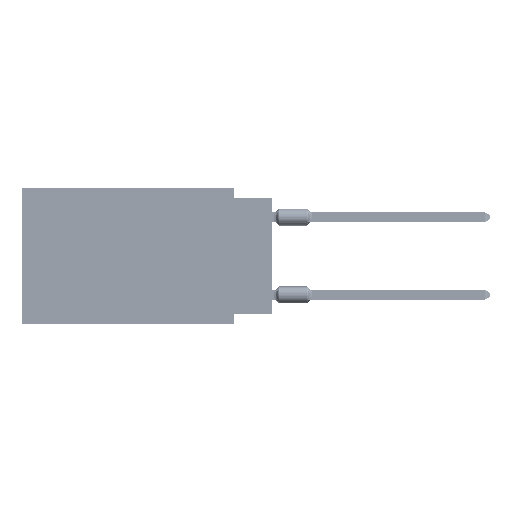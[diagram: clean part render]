
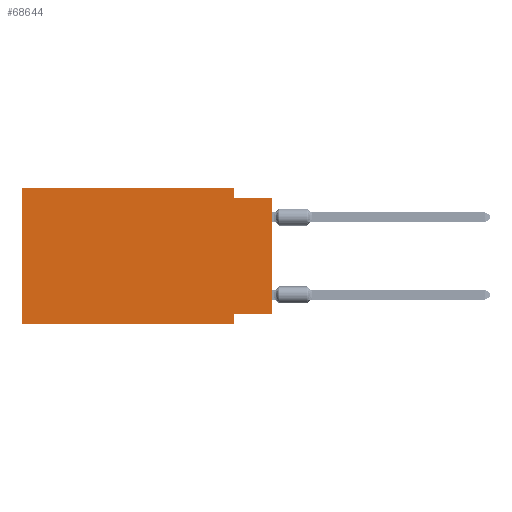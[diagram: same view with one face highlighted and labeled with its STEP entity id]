
A CAD part, left-side view. The second image highlights one B-rep face of the part: STEP entity #68644.
In plain terms, the highlighted planar face has unit normal (-1, 0, 0).
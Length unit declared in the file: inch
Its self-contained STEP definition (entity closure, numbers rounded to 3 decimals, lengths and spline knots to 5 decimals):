
#1004 = DIRECTION ( 'NONE',  ( 0., 0., 1. ) ) ;
#1669 = VECTOR ( 'NONE', #36369, 39.37008 ) ;
#2218 = EDGE_CURVE ( 'NONE', #15262, #39468, #37346, .T. ) ;
#2413 = VECTOR ( 'NONE', #67750, 39.37008 ) ;
#2530 = LINE ( 'NONE', #11505, #83795 ) ;
#3636 = VECTOR ( 'NONE', #24250, 39.37008 ) ;
#4646 = VECTOR ( 'NONE', #72819, 39.37008 ) ;
#4656 = VERTEX_POINT ( 'NONE', #49987 ) ;
#7722 = CARTESIAN_POINT ( 'NONE',  ( 0., 0., -0.025 ) ) ;
#11505 = CARTESIAN_POINT ( 'NONE',  ( 0., 0.1, 0. ) ) ;
#15262 = VERTEX_POINT ( 'NONE', #28294 ) ;
#16620 = EDGE_CURVE ( 'NONE', #43277, #98050, #51358, .T. ) ;
#16876 = VERTEX_POINT ( 'NONE', #75508 ) ;
#17993 = CARTESIAN_POINT ( 'NONE',  ( 0., 0.645, 0. ) ) ;
#18963 = ORIENTED_EDGE ( 'NONE', *, *, #16620, .T. ) ;
#24250 = DIRECTION ( 'NONE',  ( 0., -1., 0. ) ) ;
#24276 = EDGE_LOOP ( 'NONE', ( #88267, #56653, #89453, #75175, #71357, #18963, #28171, #68368 ) ) ;
#27931 = LINE ( 'NONE', #80795, #4646 ) ;
#28171 = ORIENTED_EDGE ( 'NONE', *, *, #62878, .F. ) ;
#28294 = CARTESIAN_POINT ( 'NONE',  ( 0., 0.645, 0. ) ) ;
#29452 = CARTESIAN_POINT ( 'NONE',  ( 0., 0.1, -0.325 ) ) ;
#32954 = DIRECTION ( 'NONE',  ( 0., 0., -1. ) ) ;
#32984 = DIRECTION ( 'NONE',  ( 0., 0., -1. ) ) ;
#34914 = VERTEX_POINT ( 'NONE', #29452 ) ;
#34964 = CARTESIAN_POINT ( 'NONE',  ( 0., 0.1, 0. ) ) ;
#36369 = DIRECTION ( 'NONE',  ( 0., 1., 0. ) ) ;
#37346 = LINE ( 'NONE', #92174, #2413 ) ;
#38599 = EDGE_CURVE ( 'NONE', #16876, #40599, #75107, .T. ) ;
#39468 = VERTEX_POINT ( 'NONE', #34964 ) ;
#40599 = VERTEX_POINT ( 'NONE', #7722 ) ;
#43277 = VERTEX_POINT ( 'NONE', #55944 ) ;
#43360 = CARTESIAN_POINT ( 'NONE',  ( 0., 0., -0.325 ) ) ;
#44192 = CARTESIAN_POINT ( 'NONE',  ( 0., 0., -0.025 ) ) ;
#49382 = PLANE ( 'NONE',  #57606 ) ;
#49987 = CARTESIAN_POINT ( 'NONE',  ( 0., 0., -0.325 ) ) ;
#50325 = LINE ( 'NONE', #43360, #1669 ) ;
#51358 = LINE ( 'NONE', #67307, #3636 ) ;
#52248 = VECTOR ( 'NONE', #97023, 39.37008 ) ;
#53102 = DIRECTION ( 'NONE',  ( 0., 0., -1. ) ) ;
#53448 = EDGE_CURVE ( 'NONE', #39468, #16876, #2530, .T. ) ;
#55433 = VECTOR ( 'NONE', #53102, 39.37008 ) ;
#55944 = CARTESIAN_POINT ( 'NONE',  ( 0., 0.645, -0.35 ) ) ;
#56653 = ORIENTED_EDGE ( 'NONE', *, *, #38599, .F. ) ;
#57606 = AXIS2_PLACEMENT_3D ( 'NONE', #17993, #86795, #32954 ) ;
#62878 = EDGE_CURVE ( 'NONE', #34914, #98050, #77878, .T. ) ;
#64839 = FACE_OUTER_BOUND ( 'NONE', #24276, .T. ) ;
#65180 = CARTESIAN_POINT ( 'NONE',  ( 0., 0.1, -0.35 ) ) ;
#67307 = CARTESIAN_POINT ( 'NONE',  ( 0., 0.645, -0.35 ) ) ;
#67750 = DIRECTION ( 'NONE',  ( 0., -1., 0. ) ) ;
#68368 = ORIENTED_EDGE ( 'NONE', *, *, #83327, .F. ) ;
#68644 = ADVANCED_FACE ( 'NONE', ( #64839 ), #49382, .F. ) ;
#69832 = LINE ( 'NONE', #90824, #92388 ) ;
#71357 = ORIENTED_EDGE ( 'NONE', *, *, #81735, .F. ) ;
#72819 = DIRECTION ( 'NONE',  ( 0., 0., 1. ) ) ;
#75107 = LINE ( 'NONE', #44192, #52248 ) ;
#75175 = ORIENTED_EDGE ( 'NONE', *, *, #2218, .F. ) ;
#75508 = CARTESIAN_POINT ( 'NONE',  ( 0., 0.1, -0.025 ) ) ;
#77878 = LINE ( 'NONE', #85369, #55433 ) ;
#80795 = CARTESIAN_POINT ( 'NONE',  ( 0., 0.645, 0. ) ) ;
#81735 = EDGE_CURVE ( 'NONE', #43277, #15262, #27931, .T. ) ;
#83068 = EDGE_CURVE ( 'NONE', #4656, #40599, #69832, .T. ) ;
#83327 = EDGE_CURVE ( 'NONE', #4656, #34914, #50325, .T. ) ;
#83795 = VECTOR ( 'NONE', #32984, 39.37008 ) ;
#85369 = CARTESIAN_POINT ( 'NONE',  ( 0., 0.1, -0.35 ) ) ;
#86795 = DIRECTION ( 'NONE',  ( 1., 0., 0. ) ) ;
#88267 = ORIENTED_EDGE ( 'NONE', *, *, #83068, .T. ) ;
#89453 = ORIENTED_EDGE ( 'NONE', *, *, #53448, .F. ) ;
#90824 = CARTESIAN_POINT ( 'NONE',  ( 0., 0., 0. ) ) ;
#92174 = CARTESIAN_POINT ( 'NONE',  ( 0., 0.645, 0. ) ) ;
#92388 = VECTOR ( 'NONE', #1004, 39.37008 ) ;
#97023 = DIRECTION ( 'NONE',  ( 0., -1., 0. ) ) ;
#98050 = VERTEX_POINT ( 'NONE', #65180 ) ;
